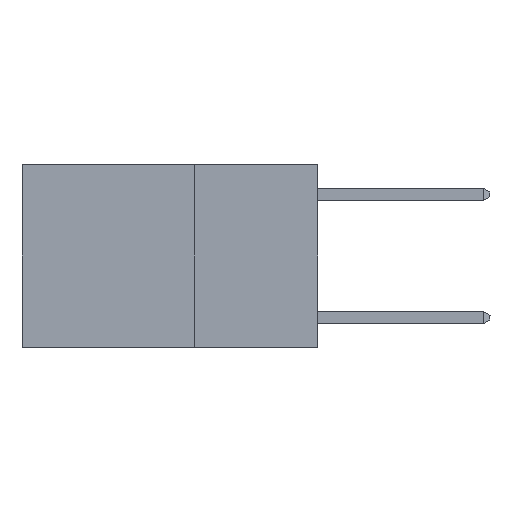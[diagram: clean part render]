
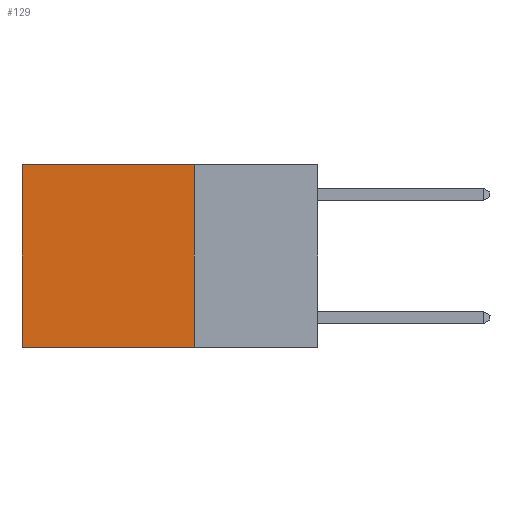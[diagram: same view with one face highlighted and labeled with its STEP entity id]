
A CAD part, left-side view. The second image highlights one B-rep face of the part: STEP entity #129.
In plain terms, the highlighted planar face has unit normal (-1, 0, 0).
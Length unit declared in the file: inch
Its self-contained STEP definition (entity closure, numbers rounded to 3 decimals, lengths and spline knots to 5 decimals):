
#129 = ADVANCED_FACE ( 'NONE', ( #10224 ), #4181, .F. ) ;
#476 = CARTESIAN_POINT ( 'NONE',  ( 0.2625, 0.25, 0. ) ) ;
#617 = VERTEX_POINT ( 'NONE', #7842 ) ;
#1059 = LINE ( 'NONE', #20751, #22050 ) ;
#4181 = PLANE ( 'NONE',  #23009 ) ;
#4628 = ORIENTED_EDGE ( 'NONE', *, *, #23166, .F. ) ;
#4687 = VECTOR ( 'NONE', #11225, 39.37008 ) ;
#5532 = LINE ( 'NONE', #13061, #22565 ) ;
#6678 = DIRECTION ( 'NONE',  ( 0., 0., -1. ) ) ;
#6900 = CARTESIAN_POINT ( 'NONE',  ( 0.2625, 0.25, 0. ) ) ;
#7477 = DIRECTION ( 'NONE',  ( 0., 0., -1. ) ) ;
#7842 = CARTESIAN_POINT ( 'NONE',  ( 0.2625, 0.25, -0.37 ) ) ;
#8851 = CARTESIAN_POINT ( 'NONE',  ( 0.2625, 0.6, 0. ) ) ;
#9577 = VERTEX_POINT ( 'NONE', #8851 ) ;
#9704 = VERTEX_POINT ( 'NONE', #21783 ) ;
#9760 = DIRECTION ( 'NONE',  ( 1., 0., 0. ) ) ;
#10224 = FACE_OUTER_BOUND ( 'NONE', #19058, .T. ) ;
#11225 = DIRECTION ( 'NONE',  ( 0., 1., 0. ) ) ;
#11402 = DIRECTION ( 'NONE',  ( 0., 0., -1. ) ) ;
#11642 = VERTEX_POINT ( 'NONE', #17748 ) ;
#12256 = VECTOR ( 'NONE', #6678, 39.37008 ) ;
#12344 = LINE ( 'NONE', #16672, #4687 ) ;
#13061 = CARTESIAN_POINT ( 'NONE',  ( 0.2625, 0.6, 0. ) ) ;
#14290 = EDGE_CURVE ( 'NONE', #9577, #9704, #5532, .T. ) ;
#15438 = DIRECTION ( 'NONE',  ( 0., 1., 0. ) ) ;
#16226 = ORIENTED_EDGE ( 'NONE', *, *, #18510, .F. ) ;
#16672 = CARTESIAN_POINT ( 'NONE',  ( 0.2625, 0.25, -0.37 ) ) ;
#17748 = CARTESIAN_POINT ( 'NONE',  ( 0.2625, 0.25, 0. ) ) ;
#18510 = EDGE_CURVE ( 'NONE', #11642, #617, #20196, .T. ) ;
#18750 = ORIENTED_EDGE ( 'NONE', *, *, #21359, .T. ) ;
#19058 = EDGE_LOOP ( 'NONE', ( #22443, #4628, #16226, #18750 ) ) ;
#20196 = LINE ( 'NONE', #6900, #12256 ) ;
#20751 = CARTESIAN_POINT ( 'NONE',  ( 0.2625, 0.25, 0. ) ) ;
#21359 = EDGE_CURVE ( 'NONE', #11642, #9577, #1059, .T. ) ;
#21783 = CARTESIAN_POINT ( 'NONE',  ( 0.2625, 0.6, -0.37 ) ) ;
#22050 = VECTOR ( 'NONE', #15438, 39.37008 ) ;
#22443 = ORIENTED_EDGE ( 'NONE', *, *, #14290, .T. ) ;
#22565 = VECTOR ( 'NONE', #7477, 39.37008 ) ;
#23009 = AXIS2_PLACEMENT_3D ( 'NONE', #476, #9760, #11402 ) ;
#23166 = EDGE_CURVE ( 'NONE', #617, #9704, #12344, .T. ) ;
